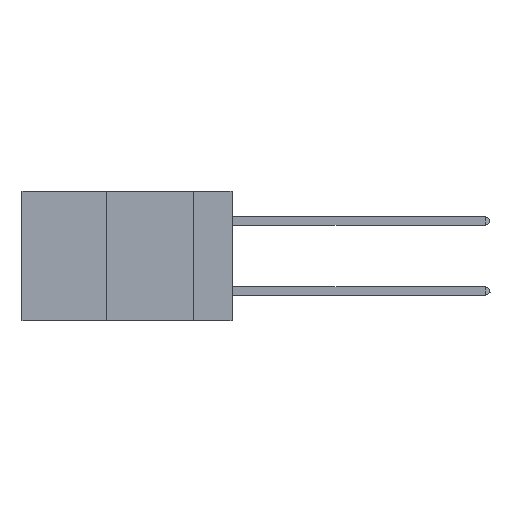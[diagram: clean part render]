
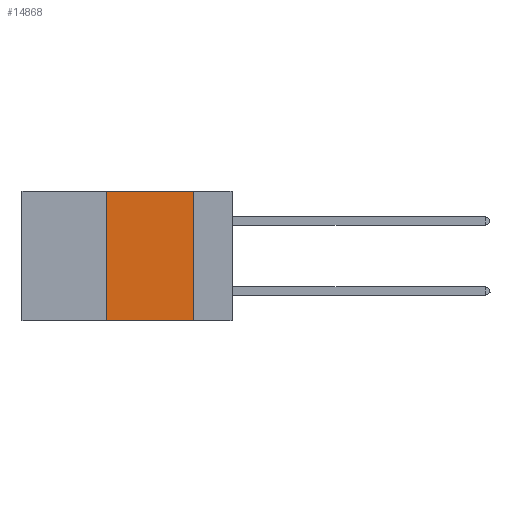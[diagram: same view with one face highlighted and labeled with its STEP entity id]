
A CAD part, left-side view. The second image highlights one B-rep face of the part: STEP entity #14868.
In plain terms, the highlighted planar face has unit normal (-1, 0, 0).
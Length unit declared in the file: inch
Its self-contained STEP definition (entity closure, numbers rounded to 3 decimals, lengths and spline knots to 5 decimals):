
#440 = LINE ( 'NONE', #4224, #13719 ) ;
#644 = DIRECTION ( 'NONE',  ( 0., -1., 0. ) ) ;
#1017 = DIRECTION ( 'NONE',  ( 1., 0., 0. ) ) ;
#1414 = ORIENTED_EDGE ( 'NONE', *, *, #8653, .F. ) ;
#2523 = DIRECTION ( 'NONE',  ( 0., 0., -1. ) ) ;
#3318 = VECTOR ( 'NONE', #644, 39.37008 ) ;
#3700 = VERTEX_POINT ( 'NONE', #20785 ) ;
#4224 = CARTESIAN_POINT ( 'NONE',  ( 0., 0.6, 0. ) ) ;
#4481 = CARTESIAN_POINT ( 'NONE',  ( 0., 0.36, 0. ) ) ;
#4797 = ORIENTED_EDGE ( 'NONE', *, *, #15935, .T. ) ;
#5352 = VERTEX_POINT ( 'NONE', #17041 ) ;
#8653 = EDGE_CURVE ( 'NONE', #3700, #10764, #16066, .T. ) ;
#9145 = CARTESIAN_POINT ( 'NONE',  ( 0., 0.6, 0. ) ) ;
#10113 = LINE ( 'NONE', #20419, #17034 ) ;
#10309 = ORIENTED_EDGE ( 'NONE', *, *, #16023, .F. ) ;
#10764 = VERTEX_POINT ( 'NONE', #16532 ) ;
#10839 = EDGE_LOOP ( 'NONE', ( #12422, #10309, #1414, #4797 ) ) ;
#11194 = VECTOR ( 'NONE', #12456, 39.37008 ) ;
#12163 = VERTEX_POINT ( 'NONE', #17111 ) ;
#12422 = ORIENTED_EDGE ( 'NONE', *, *, #18238, .F. ) ;
#12443 = DIRECTION ( 'NONE',  ( 0., 0., -1. ) ) ;
#12456 = DIRECTION ( 'NONE',  ( 0., 0., 1. ) ) ;
#13719 = VECTOR ( 'NONE', #18739, 39.37008 ) ;
#14868 = ADVANCED_FACE ( 'NONE', ( #15700 ), #15510, .F. ) ;
#15510 = PLANE ( 'NONE',  #20109 ) ;
#15700 = FACE_OUTER_BOUND ( 'NONE', #10839, .T. ) ;
#15935 = EDGE_CURVE ( 'NONE', #3700, #5352, #20344, .T. ) ;
#16023 = EDGE_CURVE ( 'NONE', #10764, #12163, #440, .T. ) ;
#16066 = LINE ( 'NONE', #4481, #11194 ) ;
#16532 = CARTESIAN_POINT ( 'NONE',  ( 0., 0.36, 0. ) ) ;
#17034 = VECTOR ( 'NONE', #12443, 39.37008 ) ;
#17041 = CARTESIAN_POINT ( 'NONE',  ( 0., 0.11, -0.37 ) ) ;
#17111 = CARTESIAN_POINT ( 'NONE',  ( 0., 0.11, 0. ) ) ;
#18238 = EDGE_CURVE ( 'NONE', #12163, #5352, #10113, .T. ) ;
#18739 = DIRECTION ( 'NONE',  ( 0., -1., 0. ) ) ;
#20109 = AXIS2_PLACEMENT_3D ( 'NONE', #9145, #1017, #2523 ) ;
#20165 = CARTESIAN_POINT ( 'NONE',  ( 0., 0.6, -0.37 ) ) ;
#20344 = LINE ( 'NONE', #20165, #3318 ) ;
#20419 = CARTESIAN_POINT ( 'NONE',  ( 0., 0.11, 0. ) ) ;
#20785 = CARTESIAN_POINT ( 'NONE',  ( 0., 0.36, -0.37 ) ) ;
